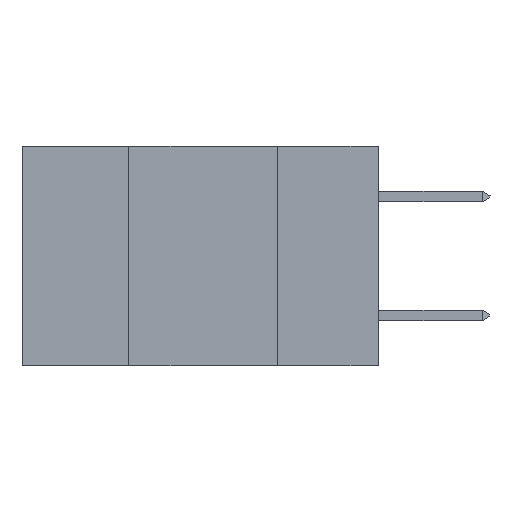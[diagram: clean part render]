
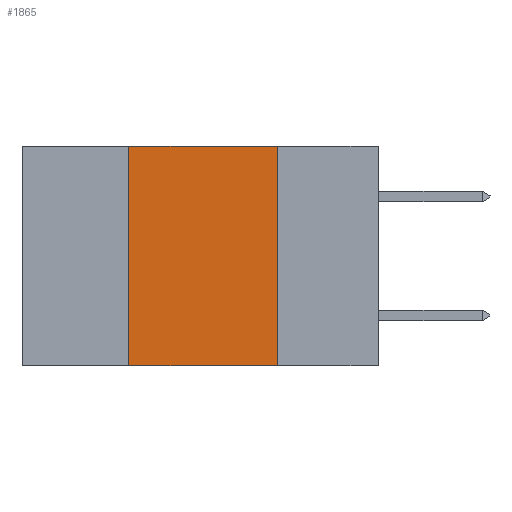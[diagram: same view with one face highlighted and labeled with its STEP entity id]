
A CAD part, left-side view. The second image highlights one B-rep face of the part: STEP entity #1865.
In plain terms, the highlighted planar face has unit normal (-1, 0, 0).
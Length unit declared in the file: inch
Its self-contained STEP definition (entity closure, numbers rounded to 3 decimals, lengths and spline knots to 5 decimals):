
#185 = PLANE ( 'NONE',  #1073 ) ;
#584 = CARTESIAN_POINT ( 'NONE',  ( 0., 0.17, -0.37 ) ) ;
#690 = DIRECTION ( 'NONE',  ( 0., -1., 0. ) ) ;
#757 = CARTESIAN_POINT ( 'NONE',  ( 0., 0.42, -0.37 ) ) ;
#946 = FACE_OUTER_BOUND ( 'NONE', #3921, .T. ) ;
#1073 = AXIS2_PLACEMENT_3D ( 'NONE', #4055, #3230, #6279 ) ;
#1380 = EDGE_CURVE ( 'NONE', #3998, #2929, #3857, .T. ) ;
#1492 = CARTESIAN_POINT ( 'NONE',  ( 0., 0.6, -0.37 ) ) ;
#1844 = VECTOR ( 'NONE', #2242, 39.37008 ) ;
#1865 = ADVANCED_FACE ( 'NONE', ( #946 ), #185, .F. ) ;
#1927 = EDGE_CURVE ( 'NONE', #5051, #6972, #6805, .T. ) ;
#1974 = CARTESIAN_POINT ( 'NONE',  ( 0., 0.17, -0.37 ) ) ;
#2109 = CARTESIAN_POINT ( 'NONE',  ( 0., 0.42, 0. ) ) ;
#2146 = ORIENTED_EDGE ( 'NONE', *, *, #1380, .F. ) ;
#2242 = DIRECTION ( 'NONE',  ( 0., 0., 1. ) ) ;
#2785 = ORIENTED_EDGE ( 'NONE', *, *, #2948, .F. ) ;
#2929 = VERTEX_POINT ( 'NONE', #6991 ) ;
#2948 = EDGE_CURVE ( 'NONE', #2929, #6972, #3514, .T. ) ;
#3194 = ORIENTED_EDGE ( 'NONE', *, *, #1927, .T. ) ;
#3230 = DIRECTION ( 'NONE',  ( 1., 0., 0. ) ) ;
#3514 = LINE ( 'NONE', #1974, #9175 ) ;
#3600 = VECTOR ( 'NONE', #9352, 39.37008 ) ;
#3857 = LINE ( 'NONE', #6879, #3600 ) ;
#3921 = EDGE_LOOP ( 'NONE', ( #2785, #2146, #6548, #3194 ) ) ;
#3998 = VERTEX_POINT ( 'NONE', #2109 ) ;
#4055 = CARTESIAN_POINT ( 'NONE',  ( 0., 0.6, 0. ) ) ;
#5051 = VERTEX_POINT ( 'NONE', #757 ) ;
#6279 = DIRECTION ( 'NONE',  ( 0., 0., -1. ) ) ;
#6410 = DIRECTION ( 'NONE',  ( 0., 0., -1. ) ) ;
#6548 = ORIENTED_EDGE ( 'NONE', *, *, #9733, .F. ) ;
#6714 = LINE ( 'NONE', #9019, #1844 ) ;
#6805 = LINE ( 'NONE', #1492, #7871 ) ;
#6879 = CARTESIAN_POINT ( 'NONE',  ( 0., 0.6, 0. ) ) ;
#6972 = VERTEX_POINT ( 'NONE', #584 ) ;
#6991 = CARTESIAN_POINT ( 'NONE',  ( 0., 0.17, 0. ) ) ;
#7871 = VECTOR ( 'NONE', #690, 39.37008 ) ;
#9019 = CARTESIAN_POINT ( 'NONE',  ( 0., 0.42, -0.37 ) ) ;
#9175 = VECTOR ( 'NONE', #6410, 39.37008 ) ;
#9352 = DIRECTION ( 'NONE',  ( 0., -1., 0. ) ) ;
#9733 = EDGE_CURVE ( 'NONE', #5051, #3998, #6714, .T. ) ;
